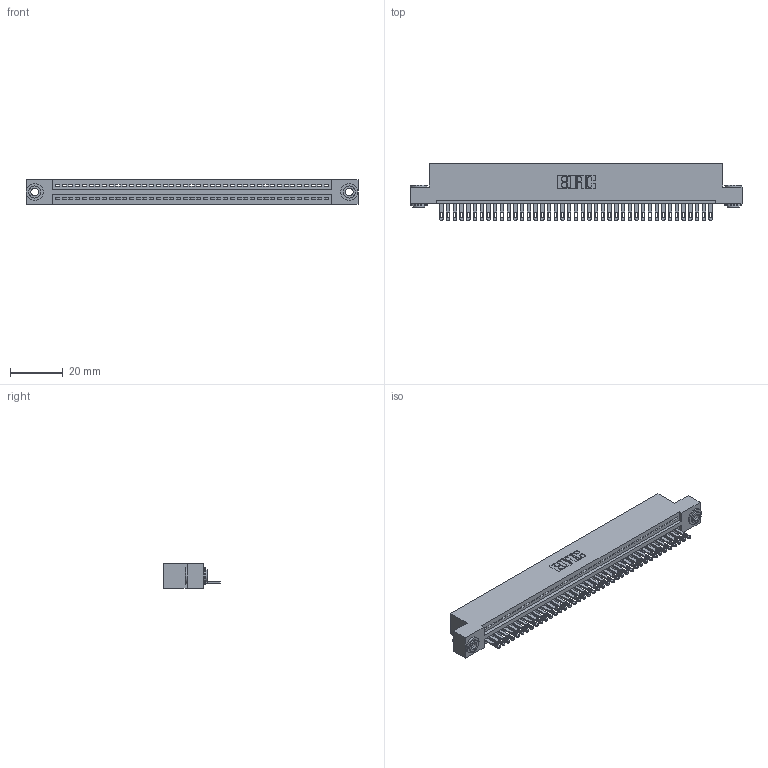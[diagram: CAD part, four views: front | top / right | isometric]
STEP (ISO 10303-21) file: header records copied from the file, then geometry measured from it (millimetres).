
FILE_DESCRIPTION (( 'STEP AP203' ), '1' );
FILE_NAME ('345-041-500-103.STEP', '2018-09-05T06:38:20', ( '' ), ( '' ), 'SwSTEP 2.0', 'SolidWorks 2016', '' );
FILE_SCHEMA (( 'CONFIG_CONTROL_DESIGN' ));
Length unit declared in the file: inch
Products named in the file (4): 345-250-002_345-250-002-102; 345-041-500-103; 345 Part_Flush Mounting Lugs - 0.156 Dia-TH; 345-292-001_345-293-100
Assembly tree (44 placements, depth 2):
  345-041-500-103
    345 Part_Flush Mounting Lugs - 0.156 Dia-TH
    345-292-001_345-293-100  x41
    345-250-002_345-250-002-102  x2
Bounding box: 125.35 x 21.51 x 9.4 mm (x, y, z)
Volume: 11942.4 mm3; surface area: 16163.3 mm2
Topology: 44 solids, 44 shells, 2378 faces, 7305 edges, 4866 vertices
Faces by surface type: plane 1484, cylinder 886, cone 8
Entity records: 31572 total; most frequent: CARTESIAN_POINT 5446, ORIENTED_EDGE 5414, DIRECTION 4791, EDGE_CURVE 2707, VECTOR 2383, LINE 2383, VERTEX_POINT 1802, AXIS2_PLACEMENT_3D 1204
